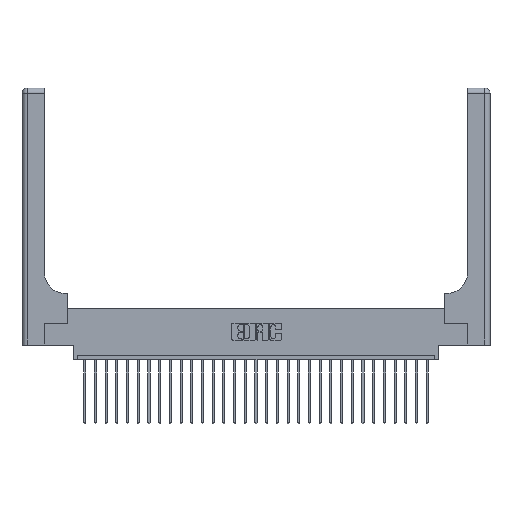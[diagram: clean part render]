
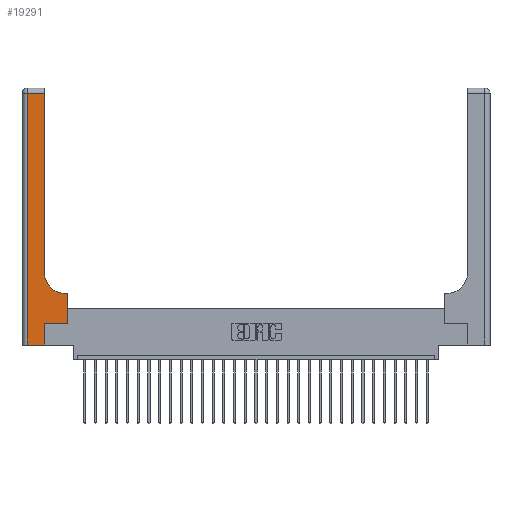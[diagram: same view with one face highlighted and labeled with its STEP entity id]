
A CAD part, top view. The second image highlights one B-rep face of the part: STEP entity #19291.
In plain terms, the highlighted planar face has unit normal (0, 0, 1).
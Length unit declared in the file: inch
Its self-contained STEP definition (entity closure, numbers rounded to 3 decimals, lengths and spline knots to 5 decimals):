
#335 = EDGE_CURVE ( 'NONE', #16565, #5409, #5271, .T. ) ;
#496 = CARTESIAN_POINT ( 'NONE',  ( 0.06, 2.94, 0.37 ) ) ;
#703 = CARTESIAN_POINT ( 'NONE',  ( 0.26, 3., 0.37 ) ) ;
#2408 = VERTEX_POINT ( 'NONE', #13831 ) ;
#2643 = VERTEX_POINT ( 'NONE', #18805 ) ;
#2738 = VECTOR ( 'NONE', #23376, 39.37008 ) ;
#3822 = CARTESIAN_POINT ( 'NONE',  ( 0.51, 0.85, 0.37 ) ) ;
#3881 = DIRECTION ( 'NONE',  ( -1., 0., 0. ) ) ;
#4247 = CARTESIAN_POINT ( 'NONE',  ( 0.528, 0.25, 0.37 ) ) ;
#4289 = AXIS2_PLACEMENT_3D ( 'NONE', #10740, #25327, #19104 ) ;
#4402 = VERTEX_POINT ( 'NONE', #15228 ) ;
#4633 = CARTESIAN_POINT ( 'NONE',  ( 0.528, 0.6, 0.37 ) ) ;
#4675 = ORIENTED_EDGE ( 'NONE', *, *, #24925, .T. ) ;
#5271 = LINE ( 'NONE', #10765, #5583 ) ;
#5379 = DIRECTION ( 'NONE',  ( 1., 0., 0. ) ) ;
#5395 = ORIENTED_EDGE ( 'NONE', *, *, #17226, .T. ) ;
#5409 = VERTEX_POINT ( 'NONE', #16887 ) ;
#5583 = VECTOR ( 'NONE', #12863, 39.37008 ) ;
#5963 = DIRECTION ( 'NONE',  ( 1., 0., 0. ) ) ;
#6010 = LINE ( 'NONE', #14263, #6344 ) ;
#6250 = ORIENTED_EDGE ( 'NONE', *, *, #23891, .T. ) ;
#6344 = VECTOR ( 'NONE', #3881, 39.37008 ) ;
#6367 = LINE ( 'NONE', #11218, #2738 ) ;
#6671 = EDGE_CURVE ( 'NONE', #2643, #24039, #6367, .T. ) ;
#7140 = EDGE_CURVE ( 'NONE', #21930, #9052, #6010, .T. ) ;
#7633 = CARTESIAN_POINT ( 'NONE',  ( 0.528, 0.25, 0.37 ) ) ;
#8109 = LINE ( 'NONE', #15444, #18519 ) ;
#8370 = LINE ( 'NONE', #703, #16818 ) ;
#8410 = CARTESIAN_POINT ( 'NONE',  ( 0.265, 0.25, 0.37 ) ) ;
#8492 = CIRCLE ( 'NONE', #8737, 0.25 ) ;
#8664 = LINE ( 'NONE', #21633, #24680 ) ;
#8737 = AXIS2_PLACEMENT_3D ( 'NONE', #3822, #18425, #5963 ) ;
#9052 = VERTEX_POINT ( 'NONE', #15177 ) ;
#9174 = VECTOR ( 'NONE', #19470, 39.37008 ) ;
#9882 = VERTEX_POINT ( 'NONE', #7633 ) ;
#10740 = CARTESIAN_POINT ( 'NONE',  ( 0., 3., 0.37 ) ) ;
#10765 = CARTESIAN_POINT ( 'NONE',  ( 0.06, 3., 0.37 ) ) ;
#11218 = CARTESIAN_POINT ( 'NONE',  ( 0.265, 0., 0.37 ) ) ;
#11483 = DIRECTION ( 'NONE',  ( 1., 0., 0. ) ) ;
#11791 = ORIENTED_EDGE ( 'NONE', *, *, #24715, .T. ) ;
#11986 = ORIENTED_EDGE ( 'NONE', *, *, #15968, .T. ) ;
#12074 = LINE ( 'NONE', #4247, #14951 ) ;
#12694 = ORIENTED_EDGE ( 'NONE', *, *, #19411, .T. ) ;
#12863 = DIRECTION ( 'NONE',  ( 0., -1., 0. ) ) ;
#13831 = CARTESIAN_POINT ( 'NONE',  ( 0.26, 2.94, 0.37 ) ) ;
#14263 = CARTESIAN_POINT ( 'NONE',  ( 0.26, 0.6, 0.37 ) ) ;
#14445 = EDGE_LOOP ( 'NONE', ( #11986, #12694, #14801, #5395, #22465, #4675, #11791, #26774, #6250 ) ) ;
#14801 = ORIENTED_EDGE ( 'NONE', *, *, #335, .T. ) ;
#14951 = VECTOR ( 'NONE', #18851, 39.37008 ) ;
#15177 = CARTESIAN_POINT ( 'NONE',  ( 0.51, 0.6, 0.37 ) ) ;
#15228 = CARTESIAN_POINT ( 'NONE',  ( 0.26, 0.85, 0.37 ) ) ;
#15444 = CARTESIAN_POINT ( 'NONE',  ( 0.265, 0.25, 0.37 ) ) ;
#15968 = EDGE_CURVE ( 'NONE', #4402, #2408, #8370, .T. ) ;
#16565 = VERTEX_POINT ( 'NONE', #496 ) ;
#16818 = VECTOR ( 'NONE', #17400, 39.37008 ) ;
#16887 = CARTESIAN_POINT ( 'NONE',  ( 0.06, 0., 0.37 ) ) ;
#17226 = EDGE_CURVE ( 'NONE', #5409, #2643, #8664, .T. ) ;
#17400 = DIRECTION ( 'NONE',  ( 0., 1., 0. ) ) ;
#18425 = DIRECTION ( 'NONE',  ( 0., 0., -1. ) ) ;
#18519 = VECTOR ( 'NONE', #11483, 39.37008 ) ;
#18805 = CARTESIAN_POINT ( 'NONE',  ( 0.265, 0., 0.37 ) ) ;
#18851 = DIRECTION ( 'NONE',  ( 0., 1., 0. ) ) ;
#19104 = DIRECTION ( 'NONE',  ( -1., 0., 0. ) ) ;
#19291 = ADVANCED_FACE ( 'NONE', ( #19620 ), #21237, .F. ) ;
#19411 = EDGE_CURVE ( 'NONE', #2408, #16565, #19961, .T. ) ;
#19470 = DIRECTION ( 'NONE',  ( -1., 0., 0. ) ) ;
#19620 = FACE_OUTER_BOUND ( 'NONE', #14445, .T. ) ;
#19961 = LINE ( 'NONE', #26061, #9174 ) ;
#21237 = PLANE ( 'NONE',  #4289 ) ;
#21633 = CARTESIAN_POINT ( 'NONE',  ( 0., 0., 0.37 ) ) ;
#21930 = VERTEX_POINT ( 'NONE', #4633 ) ;
#22465 = ORIENTED_EDGE ( 'NONE', *, *, #6671, .T. ) ;
#23376 = DIRECTION ( 'NONE',  ( 0., 1., 0. ) ) ;
#23891 = EDGE_CURVE ( 'NONE', #9052, #4402, #8492, .T. ) ;
#24039 = VERTEX_POINT ( 'NONE', #8410 ) ;
#24680 = VECTOR ( 'NONE', #5379, 39.37008 ) ;
#24715 = EDGE_CURVE ( 'NONE', #9882, #21930, #12074, .T. ) ;
#24925 = EDGE_CURVE ( 'NONE', #24039, #9882, #8109, .T. ) ;
#25327 = DIRECTION ( 'NONE',  ( 0., 0., -1. ) ) ;
#26061 = CARTESIAN_POINT ( 'NONE',  ( 0., 2.94, 0.37 ) ) ;
#26774 = ORIENTED_EDGE ( 'NONE', *, *, #7140, .T. ) ;
